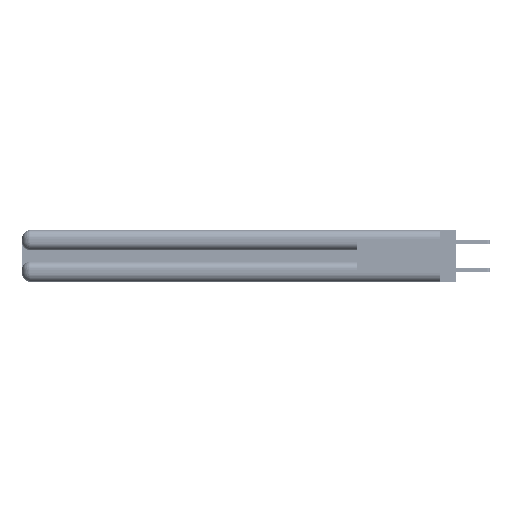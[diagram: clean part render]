
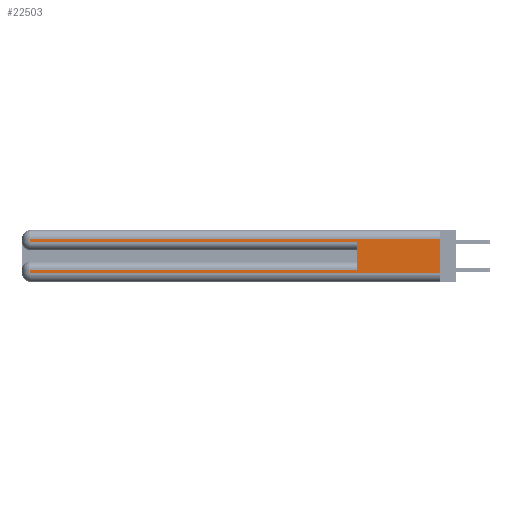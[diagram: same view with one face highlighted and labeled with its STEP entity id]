
A CAD part, left-side view. The second image highlights one B-rep face of the part: STEP entity #22503.
In plain terms, the highlighted planar face has unit normal (-1, 0, 0).
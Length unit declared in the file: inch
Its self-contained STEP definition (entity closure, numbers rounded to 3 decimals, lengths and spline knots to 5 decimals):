
#104 = CARTESIAN_POINT ( 'NONE',  ( 0., 2.94, 0.06 ) ) ;
#348 = CARTESIAN_POINT ( 'NONE',  ( 0., 2.94, 0.31 ) ) ;
#1214 = PLANE ( 'NONE',  #8971 ) ;
#1257 = CARTESIAN_POINT ( 'NONE',  ( 0., 2.94, 0.285 ) ) ;
#1274 = ORIENTED_EDGE ( 'NONE', *, *, #37415, .T. ) ;
#1513 = VECTOR ( 'NONE', #42545, 39.37008 ) ;
#2312 = VERTEX_POINT ( 'NONE', #32929 ) ;
#2380 = CARTESIAN_POINT ( 'NONE',  ( 0., 0., 0.285 ) ) ;
#6212 = VECTOR ( 'NONE', #41505, 39.37008 ) ;
#6379 = CARTESIAN_POINT ( 'NONE',  ( 0., 0., 0.06 ) ) ;
#7391 = VECTOR ( 'NONE', #18890, 39.37008 ) ;
#8600 = VERTEX_POINT ( 'NONE', #104 ) ;
#8971 = AXIS2_PLACEMENT_3D ( 'NONE', #34687, #38671, #18485 ) ;
#10223 = DIRECTION ( 'NONE',  ( 0., -1., 0. ) ) ;
#10867 = LINE ( 'NONE', #40382, #35636 ) ;
#12083 = VECTOR ( 'NONE', #10223, 39.37008 ) ;
#12552 = VERTEX_POINT ( 'NONE', #22159 ) ;
#13161 = EDGE_CURVE ( 'NONE', #12552, #24448, #10867, .T. ) ;
#13788 = ORIENTED_EDGE ( 'NONE', *, *, #20194, .T. ) ;
#15113 = ORIENTED_EDGE ( 'NONE', *, *, #50552, .T. ) ;
#15608 = VECTOR ( 'NONE', #26298, 39.37008 ) ;
#16528 = VECTOR ( 'NONE', #48175, 39.37008 ) ;
#18485 = DIRECTION ( 'NONE',  ( 0., 0., -1. ) ) ;
#18890 = DIRECTION ( 'NONE',  ( 0., 1., 0. ) ) ;
#19834 = DIRECTION ( 'NONE',  ( 0., 0., 1. ) ) ;
#20194 = EDGE_CURVE ( 'NONE', #12552, #41645, #32811, .T. ) ;
#21708 = EDGE_LOOP ( 'NONE', ( #42273, #15113, #29830, #23040, #37908, #13788, #1274, #50228 ) ) ;
#22159 = CARTESIAN_POINT ( 'NONE',  ( 0., 0.6, 0.085 ) ) ;
#22503 = ADVANCED_FACE ( 'NONE', ( #33208 ), #1214, .F. ) ;
#23040 = ORIENTED_EDGE ( 'NONE', *, *, #37606, .T. ) ;
#24448 = VERTEX_POINT ( 'NONE', #47308 ) ;
#25109 = LINE ( 'NONE', #46187, #6212 ) ;
#25589 = LINE ( 'NONE', #6379, #16528 ) ;
#26298 = DIRECTION ( 'NONE',  ( 0., 0., -1. ) ) ;
#27782 = CARTESIAN_POINT ( 'NONE',  ( 0., 0., 0.085 ) ) ;
#27870 = EDGE_CURVE ( 'NONE', #8600, #2312, #25589, .T. ) ;
#28182 = EDGE_CURVE ( 'NONE', #39002, #2312, #39904, .T. ) ;
#28751 = VECTOR ( 'NONE', #51934, 39.37008 ) ;
#29830 = ORIENTED_EDGE ( 'NONE', *, *, #47033, .T. ) ;
#32666 = LINE ( 'NONE', #34721, #28751 ) ;
#32811 = LINE ( 'NONE', #27782, #7391 ) ;
#32929 = CARTESIAN_POINT ( 'NONE',  ( 0., 0., 0.06 ) ) ;
#33208 = FACE_OUTER_BOUND ( 'NONE', #21708, .T. ) ;
#34132 = CARTESIAN_POINT ( 'NONE',  ( 0., 0., 0.31 ) ) ;
#34687 = CARTESIAN_POINT ( 'NONE',  ( 0., 0., 0.37 ) ) ;
#34721 = CARTESIAN_POINT ( 'NONE',  ( 0., 0., 0.31 ) ) ;
#35205 = CARTESIAN_POINT ( 'NONE',  ( 0., 2.94, 0.37 ) ) ;
#35636 = VECTOR ( 'NONE', #19834, 39.37008 ) ;
#37415 = EDGE_CURVE ( 'NONE', #41645, #8600, #25109, .T. ) ;
#37606 = EDGE_CURVE ( 'NONE', #38323, #24448, #49774, .T. ) ;
#37908 = ORIENTED_EDGE ( 'NONE', *, *, #13161, .F. ) ;
#38323 = VERTEX_POINT ( 'NONE', #1257 ) ;
#38671 = DIRECTION ( 'NONE',  ( 1., 0., 0. ) ) ;
#39002 = VERTEX_POINT ( 'NONE', #34132 ) ;
#39904 = LINE ( 'NONE', #41999, #1513 ) ;
#40382 = CARTESIAN_POINT ( 'NONE',  ( 0., 0.6, 0.145 ) ) ;
#41505 = DIRECTION ( 'NONE',  ( 0., 0., -1. ) ) ;
#41645 = VERTEX_POINT ( 'NONE', #51032 ) ;
#41999 = CARTESIAN_POINT ( 'NONE',  ( 0., 0., 0.37 ) ) ;
#42273 = ORIENTED_EDGE ( 'NONE', *, *, #28182, .F. ) ;
#42545 = DIRECTION ( 'NONE',  ( 0., 0., -1. ) ) ;
#46187 = CARTESIAN_POINT ( 'NONE',  ( 0., 2.94, 0.37 ) ) ;
#47033 = EDGE_CURVE ( 'NONE', #52497, #38323, #48095, .T. ) ;
#47308 = CARTESIAN_POINT ( 'NONE',  ( 0., 0.6, 0.285 ) ) ;
#48095 = LINE ( 'NONE', #35205, #15608 ) ;
#48175 = DIRECTION ( 'NONE',  ( 0., -1., 0. ) ) ;
#49774 = LINE ( 'NONE', #2380, #12083 ) ;
#50228 = ORIENTED_EDGE ( 'NONE', *, *, #27870, .T. ) ;
#50552 = EDGE_CURVE ( 'NONE', #39002, #52497, #32666, .T. ) ;
#51032 = CARTESIAN_POINT ( 'NONE',  ( 0., 2.94, 0.085 ) ) ;
#51934 = DIRECTION ( 'NONE',  ( 0., 1., 0. ) ) ;
#52497 = VERTEX_POINT ( 'NONE', #348 ) ;
